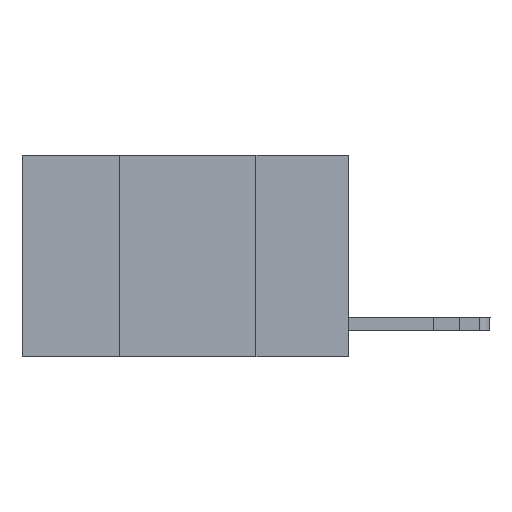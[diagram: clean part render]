
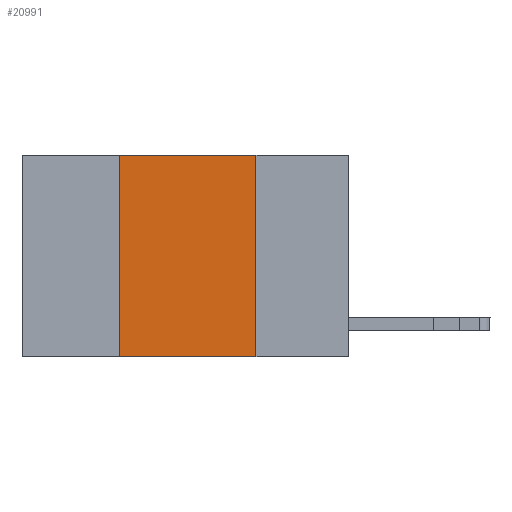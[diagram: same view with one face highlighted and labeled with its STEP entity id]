
A CAD part, left-side view. The second image highlights one B-rep face of the part: STEP entity #20991.
In plain terms, the highlighted planar face has unit normal (-1, 0, 0).
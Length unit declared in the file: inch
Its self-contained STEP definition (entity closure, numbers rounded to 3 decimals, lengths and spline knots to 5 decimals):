
#1832 = LINE ( 'NONE', #15922, #20087 ) ;
#2078 = EDGE_CURVE ( 'NONE', #4066, #17705, #9888, .T. ) ;
#4066 = VERTEX_POINT ( 'NONE', #13364 ) ;
#5074 = CARTESIAN_POINT ( 'NONE',  ( 0., 0.17, 0. ) ) ;
#5121 = LINE ( 'NONE', #6947, #9709 ) ;
#5315 = VECTOR ( 'NONE', #8150, 39.37008 ) ;
#5672 = DIRECTION ( 'NONE',  ( 0., -1., 0. ) ) ;
#6931 = ORIENTED_EDGE ( 'NONE', *, *, #2078, .F. ) ;
#6947 = CARTESIAN_POINT ( 'NONE',  ( 0., 0.17, 0. ) ) ;
#6949 = ORIENTED_EDGE ( 'NONE', *, *, #18457, .F. ) ;
#8150 = DIRECTION ( 'NONE',  ( 0., -1., 0. ) ) ;
#8168 = CARTESIAN_POINT ( 'NONE',  ( 0., 0.6, 0. ) ) ;
#8345 = PLANE ( 'NONE',  #19207 ) ;
#8755 = CARTESIAN_POINT ( 'NONE',  ( 0., 0.42, 0. ) ) ;
#9709 = VECTOR ( 'NONE', #15462, 39.37008 ) ;
#9888 = LINE ( 'NONE', #8168, #5315 ) ;
#10077 = DIRECTION ( 'NONE',  ( 1., 0., 0. ) ) ;
#10465 = ORIENTED_EDGE ( 'NONE', *, *, #11800, .T. ) ;
#10890 = EDGE_CURVE ( 'NONE', #21878, #4066, #11516, .T. ) ;
#11516 = LINE ( 'NONE', #8755, #15502 ) ;
#11711 = FACE_OUTER_BOUND ( 'NONE', #15355, .T. ) ;
#11800 = EDGE_CURVE ( 'NONE', #21878, #18475, #1832, .T. ) ;
#12108 = ORIENTED_EDGE ( 'NONE', *, *, #10890, .F. ) ;
#13364 = CARTESIAN_POINT ( 'NONE',  ( 0., 0.42, 0. ) ) ;
#15148 = CARTESIAN_POINT ( 'NONE',  ( 0., 0.6, 0. ) ) ;
#15355 = EDGE_LOOP ( 'NONE', ( #6949, #6931, #12108, #10465 ) ) ;
#15462 = DIRECTION ( 'NONE',  ( 0., 0., -1. ) ) ;
#15502 = VECTOR ( 'NONE', #19055, 39.37008 ) ;
#15529 = CARTESIAN_POINT ( 'NONE',  ( 0., 0.17, -0.37 ) ) ;
#15922 = CARTESIAN_POINT ( 'NONE',  ( 0., 0.6, -0.37 ) ) ;
#17705 = VERTEX_POINT ( 'NONE', #5074 ) ;
#18457 = EDGE_CURVE ( 'NONE', #17705, #18475, #5121, .T. ) ;
#18475 = VERTEX_POINT ( 'NONE', #15529 ) ;
#19055 = DIRECTION ( 'NONE',  ( 0., 0., 1. ) ) ;
#19207 = AXIS2_PLACEMENT_3D ( 'NONE', #15148, #10077, #22099 ) ;
#19348 = CARTESIAN_POINT ( 'NONE',  ( 0., 0.42, -0.37 ) ) ;
#20087 = VECTOR ( 'NONE', #5672, 39.37008 ) ;
#20991 = ADVANCED_FACE ( 'NONE', ( #11711 ), #8345, .F. ) ;
#21878 = VERTEX_POINT ( 'NONE', #19348 ) ;
#22099 = DIRECTION ( 'NONE',  ( 0., 0., -1. ) ) ;
